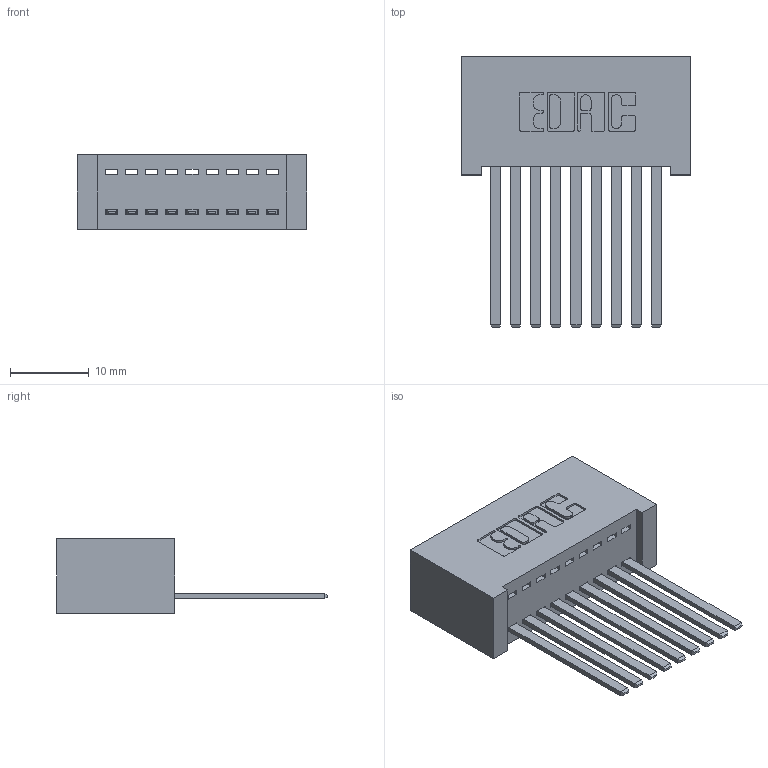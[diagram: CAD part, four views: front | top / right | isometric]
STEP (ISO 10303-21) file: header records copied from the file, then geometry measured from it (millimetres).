
FILE_DESCRIPTION (( 'STEP AP203' ), '1' );
FILE_NAME ('342-009-544-101.STEP', '2019-10-01T13:33:46', ( '' ), ( '' ), 'SwSTEP 2.0', 'SolidWorks 2016', '' );
FILE_SCHEMA (( 'CONFIG_CONTROL_DESIGN' ));
Length unit declared in the file: inch
Products named in the file (3): 342 Part_Lugless; 345-292-001_345-293-144; 342-009-544-101
Assembly tree (10 placements, depth 2):
  342-009-544-101
    342 Part_Lugless
    345-292-001_345-293-144  x9
Bounding box: 29.11 x 34.3 x 9.4 mm (x, y, z)
Volume: 2943.9 mm3; surface area: 4326.7 mm2
Topology: 10 solids, 10 shells, 570 faces, 1697 edges, 1118 vertices
Faces by surface type: plane 404, cylinder 166
Entity records: 9177 total; most frequent: CARTESIAN_POINT 1593, ORIENTED_EDGE 1538, DIRECTION 1399, EDGE_CURVE 769, LINE 653, VECTOR 653, VERTEX_POINT 510, AXIS2_PLACEMENT_3D 373
